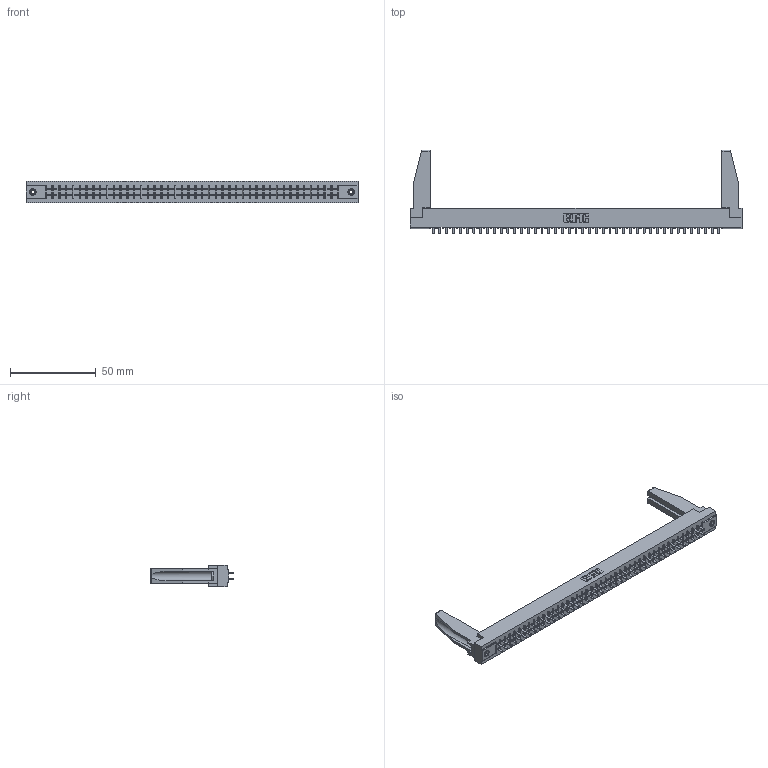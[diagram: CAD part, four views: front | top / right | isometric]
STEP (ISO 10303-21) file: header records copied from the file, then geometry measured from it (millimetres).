
FILE_DESCRIPTION (( 'STEP AP203' ), '1' );
FILE_NAME ('315-086-521-278.STEP', '2019-09-11T00:20:25', ( '' ), ( '' ), 'SwSTEP 2.0', 'SolidWorks 2016', '' );
FILE_SCHEMA (( 'CONFIG_CONTROL_DESIGN' ));
Length unit declared in the file: inch
Products named in the file (5): 305-290-001_521; 307-220-078; 345-250-001_345-250-001-102; 315-086-521-278; 305 Part_.156 Dia
Assembly tree (91 placements, depth 2):
  315-086-521-278
    305 Part_.156 Dia
    305-290-001_521  x86
    345-250-001_345-250-001-102  x2
    307-220-078  x2
Bounding box: 193.4 x 48.9 x 12.7 mm (x, y, z)
Volume: 24096.4 mm3; surface area: 29014.5 mm2
Topology: 91 solids, 91 shells, 4202 faces, 11955 edges, 7730 vertices
Faces by surface type: plane 2474, cylinder 1540, sphere 172, cone 12, torus 4
Entity records: 48755 total; most frequent: CARTESIAN_POINT 8073, ORIENTED_EDGE 7972, DIRECTION 7766, EDGE_CURVE 3986, VECTOR 3224, LINE 3224, VERTEX_POINT 2536, AXIS2_PLACEMENT_3D 2271
